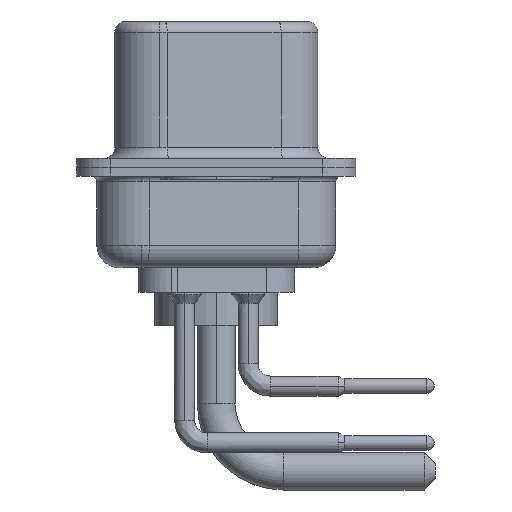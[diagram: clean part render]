
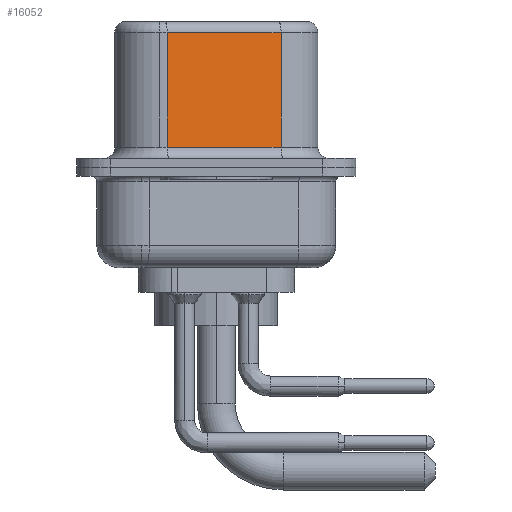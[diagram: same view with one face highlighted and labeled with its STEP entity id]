
A CAD part, left-side view. The second image highlights one B-rep face of the part: STEP entity #16052.
In plain terms, the highlighted planar face has unit normal (-0.985, -0.174, 0).
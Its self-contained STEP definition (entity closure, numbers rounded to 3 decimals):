
#550 = ORIENTED_EDGE ( 'NONE', *, *, #1327, .F. ) ;
#955 = CARTESIAN_POINT ( 'NONE',  ( 4.58, -2.897, 0.9 ) ) ;
#1078 = LINE ( 'NONE', #955, #11272 ) ;
#1327 = EDGE_CURVE ( 'NONE', #7338, #12406, #8054, .T. ) ;
#1691 = AXIS2_PLACEMENT_3D ( 'NONE', #14346, #8614, #10204 ) ;
#2495 = ORIENTED_EDGE ( 'NONE', *, *, #20101, .T. ) ;
#3466 = CARTESIAN_POINT ( 'NONE',  ( 4.58, -2.897, 6.02 ) ) ;
#6254 = CARTESIAN_POINT ( 'NONE',  ( 4.58, -2.897, 0.9 ) ) ;
#6388 = CARTESIAN_POINT ( 'NONE',  ( 4.58, -2.897, 6.02 ) ) ;
#6812 = DIRECTION ( 'NONE',  ( 0., 0., -1. ) ) ;
#6835 = CARTESIAN_POINT ( 'NONE',  ( 3.68, 2.203, 0.9 ) ) ;
#6910 = PLANE ( 'NONE',  #1691 ) ;
#7338 = VERTEX_POINT ( 'NONE', #6388 ) ;
#8054 = LINE ( 'NONE', #9636, #9244 ) ;
#8614 = DIRECTION ( 'NONE',  ( 0.985, 0.174, 0. ) ) ;
#9244 = VECTOR ( 'NONE', #15129, 1000. ) ;
#9636 = CARTESIAN_POINT ( 'NONE',  ( 4.58, -2.897, 6.52 ) ) ;
#10204 = DIRECTION ( 'NONE',  ( -0.174, 0.985, 0. ) ) ;
#10427 = CARTESIAN_POINT ( 'NONE',  ( 3.68, 2.203, 6.02 ) ) ;
#10699 = FACE_OUTER_BOUND ( 'NONE', #13717, .T. ) ;
#11272 = VECTOR ( 'NONE', #16315, 1000. ) ;
#11375 = ORIENTED_EDGE ( 'NONE', *, *, #12924, .T. ) ;
#11966 = VERTEX_POINT ( 'NONE', #10427 ) ;
#12406 = VERTEX_POINT ( 'NONE', #6254 ) ;
#12702 = ORIENTED_EDGE ( 'NONE', *, *, #19499, .T. ) ;
#12924 = EDGE_CURVE ( 'NONE', #14269, #12406, #1078, .T. ) ;
#13717 = EDGE_LOOP ( 'NONE', ( #550, #12702, #2495, #11375 ) ) ;
#14269 = VERTEX_POINT ( 'NONE', #6835 ) ;
#14346 = CARTESIAN_POINT ( 'NONE',  ( 4.58, -2.897, 6.52 ) ) ;
#15129 = DIRECTION ( 'NONE',  ( 0., 0., -1. ) ) ;
#15960 = LINE ( 'NONE', #16082, #23292 ) ;
#16052 = ADVANCED_FACE ( 'NONE', ( #10699 ), #6910, .F. ) ;
#16082 = CARTESIAN_POINT ( 'NONE',  ( 3.68, 2.203, 6.52 ) ) ;
#16264 = LINE ( 'NONE', #3466, #17106 ) ;
#16315 = DIRECTION ( 'NONE',  ( 0.174, -0.985, 0. ) ) ;
#17106 = VECTOR ( 'NONE', #23546, 1000. ) ;
#19499 = EDGE_CURVE ( 'NONE', #7338, #11966, #16264, .T. ) ;
#20101 = EDGE_CURVE ( 'NONE', #11966, #14269, #15960, .T. ) ;
#23292 = VECTOR ( 'NONE', #6812, 1000. ) ;
#23546 = DIRECTION ( 'NONE',  ( -0.174, 0.985, 0. ) ) ;
